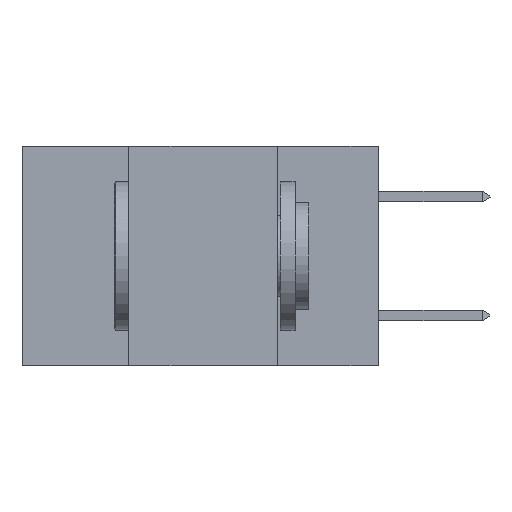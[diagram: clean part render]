
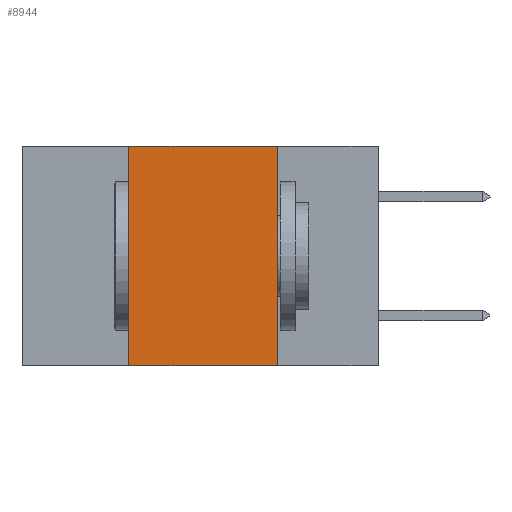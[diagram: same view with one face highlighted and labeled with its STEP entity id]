
A CAD part, left-side view. The second image highlights one B-rep face of the part: STEP entity #8944.
In plain terms, the highlighted planar face has unit normal (-1, 0, 0).
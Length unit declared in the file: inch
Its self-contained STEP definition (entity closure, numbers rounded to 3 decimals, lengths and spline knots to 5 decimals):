
#418 = CARTESIAN_POINT ( 'NONE',  ( 0., 0.42, -0.37 ) ) ;
#821 = CARTESIAN_POINT ( 'NONE',  ( 0., 0.6, 0. ) ) ;
#1214 = FACE_OUTER_BOUND ( 'NONE', #7747, .T. ) ;
#1355 = EDGE_CURVE ( 'NONE', #9632, #8964, #11382, .T. ) ;
#1765 = LINE ( 'NONE', #10052, #10947 ) ;
#2519 = DIRECTION ( 'NONE',  ( 0., 0., -1. ) ) ;
#2670 = EDGE_CURVE ( 'NONE', #9632, #7191, #11208, .T. ) ;
#3121 = VECTOR ( 'NONE', #11436, 39.37008 ) ;
#3570 = DIRECTION ( 'NONE',  ( 1., 0., 0. ) ) ;
#3832 = DIRECTION ( 'NONE',  ( 0., 0., 1. ) ) ;
#4078 = EDGE_CURVE ( 'NONE', #8964, #7564, #6469, .T. ) ;
#4389 = DIRECTION ( 'NONE',  ( 0., -1., 0. ) ) ;
#4433 = VECTOR ( 'NONE', #3832, 39.37008 ) ;
#4616 = CARTESIAN_POINT ( 'NONE',  ( 0., 0.42, 0. ) ) ;
#5289 = AXIS2_PLACEMENT_3D ( 'NONE', #821, #3570, #2519 ) ;
#5554 = DIRECTION ( 'NONE',  ( 0., 0., -1. ) ) ;
#6130 = CARTESIAN_POINT ( 'NONE',  ( 0., 0.6, -0.37 ) ) ;
#6469 = LINE ( 'NONE', #9490, #3121 ) ;
#6720 = ORIENTED_EDGE ( 'NONE', *, *, #9757, .F. ) ;
#7050 = CARTESIAN_POINT ( 'NONE',  ( 0., 0.42, 0. ) ) ;
#7191 = VERTEX_POINT ( 'NONE', #10527 ) ;
#7564 = VERTEX_POINT ( 'NONE', #8333 ) ;
#7747 = EDGE_LOOP ( 'NONE', ( #6720, #11364, #8482, #8390 ) ) ;
#8333 = CARTESIAN_POINT ( 'NONE',  ( 0., 0.17, 0. ) ) ;
#8390 = ORIENTED_EDGE ( 'NONE', *, *, #2670, .T. ) ;
#8482 = ORIENTED_EDGE ( 'NONE', *, *, #1355, .F. ) ;
#8944 = ADVANCED_FACE ( 'NONE', ( #1214 ), #11440, .F. ) ;
#8964 = VERTEX_POINT ( 'NONE', #7050 ) ;
#9490 = CARTESIAN_POINT ( 'NONE',  ( 0., 0.6, 0. ) ) ;
#9632 = VERTEX_POINT ( 'NONE', #418 ) ;
#9757 = EDGE_CURVE ( 'NONE', #7564, #7191, #1765, .T. ) ;
#10052 = CARTESIAN_POINT ( 'NONE',  ( 0., 0.17, 0. ) ) ;
#10486 = VECTOR ( 'NONE', #4389, 39.37008 ) ;
#10527 = CARTESIAN_POINT ( 'NONE',  ( 0., 0.17, -0.37 ) ) ;
#10947 = VECTOR ( 'NONE', #5554, 39.37008 ) ;
#11208 = LINE ( 'NONE', #6130, #10486 ) ;
#11364 = ORIENTED_EDGE ( 'NONE', *, *, #4078, .F. ) ;
#11382 = LINE ( 'NONE', #4616, #4433 ) ;
#11436 = DIRECTION ( 'NONE',  ( 0., -1., 0. ) ) ;
#11440 = PLANE ( 'NONE',  #5289 ) ;
